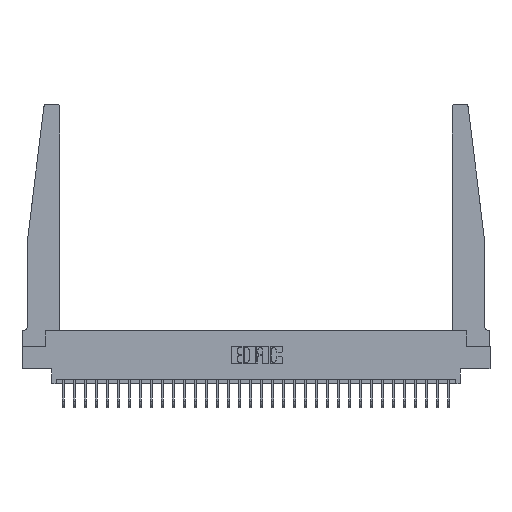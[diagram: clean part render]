
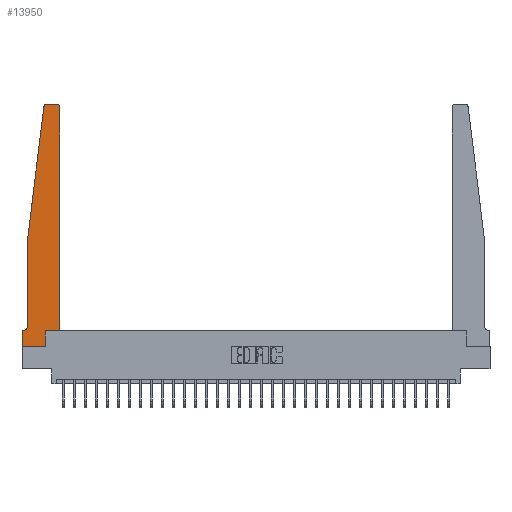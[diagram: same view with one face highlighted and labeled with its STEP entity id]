
A CAD part, top view. The second image highlights one B-rep face of the part: STEP entity #13950.
In plain terms, the highlighted planar face has unit normal (0, 0, 1).
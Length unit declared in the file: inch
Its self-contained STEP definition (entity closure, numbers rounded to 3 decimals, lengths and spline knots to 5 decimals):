
#198 = LINE ( 'NONE', #17417, #5958 ) ;
#226 = LINE ( 'NONE', #15857, #4949 ) ;
#667 = VECTOR ( 'NONE', #9376, 39.37008 ) ;
#750 = CARTESIAN_POINT ( 'NONE',  ( 0.065, 1.25, 0.37 ) ) ;
#854 = CARTESIAN_POINT ( 'NONE',  ( 0.27653, 2.72, 0.37 ) ) ;
#1331 = DIRECTION ( 'NONE',  ( 0., 1., 0. ) ) ;
#1550 = VERTEX_POINT ( 'NONE', #25755 ) ;
#1827 = CIRCLE ( 'NONE', #17989, 0.03 ) ;
#1895 = LINE ( 'NONE', #8431, #2911 ) ;
#2248 = VERTEX_POINT ( 'NONE', #2854 ) ;
#2388 = EDGE_LOOP ( 'NONE', ( #16379, #17962, #22868, #16298, #4187, #12979, #7939, #10421, #23829, #5832, #13279, #14487 ) ) ;
#2640 = AXIS2_PLACEMENT_3D ( 'NONE', #854, #18647, #5355 ) ;
#2854 = CARTESIAN_POINT ( 'NONE',  ( 0.2605, 0.18, 0.37 ) ) ;
#2911 = VECTOR ( 'NONE', #1331, 39.37008 ) ;
#3082 = DIRECTION ( 'NONE',  ( -0.122, -0.992, 0. ) ) ;
#3634 = AXIS2_PLACEMENT_3D ( 'NONE', #10922, #4018, #17439 ) ;
#3909 = EDGE_CURVE ( 'NONE', #10208, #19632, #226, .T. ) ;
#4018 = DIRECTION ( 'NONE',  ( 0., 0., 1. ) ) ;
#4091 = VERTEX_POINT ( 'NONE', #23505 ) ;
#4162 = FACE_OUTER_BOUND ( 'NONE', #2388, .T. ) ;
#4187 = ORIENTED_EDGE ( 'NONE', *, *, #14019, .T. ) ;
#4772 = VERTEX_POINT ( 'NONE', #25900 ) ;
#4949 = VECTOR ( 'NONE', #11215, 39.37008 ) ;
#5355 = DIRECTION ( 'NONE',  ( 1., 0., 0. ) ) ;
#5832 = ORIENTED_EDGE ( 'NONE', *, *, #8914, .T. ) ;
#5921 = VECTOR ( 'NONE', #16745, 39.37008 ) ;
#5958 = VECTOR ( 'NONE', #17986, 39.37008 ) ;
#6301 = VECTOR ( 'NONE', #27481, 39.37008 ) ;
#6758 = DIRECTION ( 'NONE',  ( -1., 0., 0. ) ) ;
#7132 = EDGE_CURVE ( 'NONE', #24352, #4091, #22623, .T. ) ;
#7229 = CARTESIAN_POINT ( 'NONE',  ( 0.015, 0.1875, 0.37 ) ) ;
#7259 = CARTESIAN_POINT ( 'NONE',  ( 0.395, 2.75, 0.37 ) ) ;
#7845 = DIRECTION ( 'NONE',  ( 0., 0., 1. ) ) ;
#7939 = ORIENTED_EDGE ( 'NONE', *, *, #3909, .T. ) ;
#8269 = EDGE_CURVE ( 'NONE', #19632, #15771, #9954, .T. ) ;
#8271 = CARTESIAN_POINT ( 'NONE',  ( 0., 0.1875, 0.37 ) ) ;
#8431 = CARTESIAN_POINT ( 'NONE',  ( 0.425, 0.18, 0.37 ) ) ;
#8697 = VECTOR ( 'NONE', #9607, 39.37008 ) ;
#8860 = CARTESIAN_POINT ( 'NONE',  ( 0.2605, 0., 0.37 ) ) ;
#8914 = EDGE_CURVE ( 'NONE', #2248, #9975, #198, .T. ) ;
#9376 = DIRECTION ( 'NONE',  ( -1., 0., 0. ) ) ;
#9517 = LINE ( 'NONE', #20634, #667 ) ;
#9607 = DIRECTION ( 'NONE',  ( 0., -1., 0. ) ) ;
#9949 = CARTESIAN_POINT ( 'NONE',  ( 0.25, 2.75, 0.37 ) ) ;
#9954 = LINE ( 'NONE', #16896, #21324 ) ;
#9975 = VERTEX_POINT ( 'NONE', #16059 ) ;
#10208 = VERTEX_POINT ( 'NONE', #8271 ) ;
#10421 = ORIENTED_EDGE ( 'NONE', *, *, #8269, .T. ) ;
#10436 = CARTESIAN_POINT ( 'NONE',  ( 0., 0., 0.37 ) ) ;
#10745 = VERTEX_POINT ( 'NONE', #23469 ) ;
#10922 = CARTESIAN_POINT ( 'NONE',  ( 0., 0.1875, 0.37 ) ) ;
#11215 = DIRECTION ( 'NONE',  ( 0., -1., 0. ) ) ;
#12780 = EDGE_CURVE ( 'NONE', #1550, #24352, #15119, .T. ) ;
#12979 = ORIENTED_EDGE ( 'NONE', *, *, #23203, .T. ) ;
#13062 = EDGE_CURVE ( 'NONE', #26908, #1550, #27719, .T. ) ;
#13259 = EDGE_CURVE ( 'NONE', #4091, #10745, #13395, .T. ) ;
#13279 = ORIENTED_EDGE ( 'NONE', *, *, #20565, .T. ) ;
#13395 = LINE ( 'NONE', #750, #8697 ) ;
#13950 = ADVANCED_FACE ( 'NONE', ( #4162 ), #24375, .T. ) ;
#14019 = EDGE_CURVE ( 'NONE', #10745, #27191, #23965, .T. ) ;
#14054 = CARTESIAN_POINT ( 'NONE',  ( 0.065, 1.25, 0.37 ) ) ;
#14487 = ORIENTED_EDGE ( 'NONE', *, *, #15332, .T. ) ;
#15119 = CIRCLE ( 'NONE', #2640, 0.03 ) ;
#15332 = EDGE_CURVE ( 'NONE', #4772, #26908, #1827, .T. ) ;
#15428 = CARTESIAN_POINT ( 'NONE',  ( 0.015, 0.2375, 0.37 ) ) ;
#15771 = VERTEX_POINT ( 'NONE', #8860 ) ;
#15857 = CARTESIAN_POINT ( 'NONE',  ( 0., 0., 0.37 ) ) ;
#16059 = CARTESIAN_POINT ( 'NONE',  ( 0.425, 0.18, 0.37 ) ) ;
#16298 = ORIENTED_EDGE ( 'NONE', *, *, #13259, .T. ) ;
#16379 = ORIENTED_EDGE ( 'NONE', *, *, #13062, .T. ) ;
#16444 = VECTOR ( 'NONE', #3082, 39.37008 ) ;
#16643 = DIRECTION ( 'NONE',  ( 1., 0., 0. ) ) ;
#16745 = DIRECTION ( 'NONE',  ( -1., 0., 0. ) ) ;
#16896 = CARTESIAN_POINT ( 'NONE',  ( 0., 0., 0.37 ) ) ;
#17417 = CARTESIAN_POINT ( 'NONE',  ( 0.425, 0.18, 0.37 ) ) ;
#17439 = DIRECTION ( 'NONE',  ( 1., 0., 0. ) ) ;
#17479 = AXIS2_PLACEMENT_3D ( 'NONE', #15428, #24225, #6758 ) ;
#17962 = ORIENTED_EDGE ( 'NONE', *, *, #12780, .T. ) ;
#17986 = DIRECTION ( 'NONE',  ( 1., 0., 0. ) ) ;
#17989 = AXIS2_PLACEMENT_3D ( 'NONE', #18797, #7845, #16643 ) ;
#18647 = DIRECTION ( 'NONE',  ( 0., 0., 1. ) ) ;
#18660 = CARTESIAN_POINT ( 'NONE',  ( 0.2605, 0.18, 0.37 ) ) ;
#18797 = CARTESIAN_POINT ( 'NONE',  ( 0.395, 2.72, 0.37 ) ) ;
#19632 = VERTEX_POINT ( 'NONE', #10436 ) ;
#20565 = EDGE_CURVE ( 'NONE', #9975, #4772, #1895, .T. ) ;
#20634 = CARTESIAN_POINT ( 'NONE',  ( 0.065, 0.1875, 0.37 ) ) ;
#20834 = LINE ( 'NONE', #18660, #6301 ) ;
#21324 = VECTOR ( 'NONE', #27728, 39.37008 ) ;
#22623 = LINE ( 'NONE', #14054, #16444 ) ;
#22868 = ORIENTED_EDGE ( 'NONE', *, *, #7132, .T. ) ;
#23203 = EDGE_CURVE ( 'NONE', #27191, #10208, #9517, .T. ) ;
#23469 = CARTESIAN_POINT ( 'NONE',  ( 0.065, 0.2375, 0.37 ) ) ;
#23505 = CARTESIAN_POINT ( 'NONE',  ( 0.065, 1.25, 0.37 ) ) ;
#23829 = ORIENTED_EDGE ( 'NONE', *, *, #26992, .T. ) ;
#23965 = CIRCLE ( 'NONE', #17479, 0.05 ) ;
#24225 = DIRECTION ( 'NONE',  ( 0., 0., -1. ) ) ;
#24352 = VERTEX_POINT ( 'NONE', #27952 ) ;
#24375 = PLANE ( 'NONE',  #3634 ) ;
#25755 = CARTESIAN_POINT ( 'NONE',  ( 0.27653, 2.75, 0.37 ) ) ;
#25900 = CARTESIAN_POINT ( 'NONE',  ( 0.425, 2.72, 0.37 ) ) ;
#26908 = VERTEX_POINT ( 'NONE', #7259 ) ;
#26992 = EDGE_CURVE ( 'NONE', #15771, #2248, #20834, .T. ) ;
#27191 = VERTEX_POINT ( 'NONE', #7229 ) ;
#27481 = DIRECTION ( 'NONE',  ( 0., 1., 0. ) ) ;
#27719 = LINE ( 'NONE', #9949, #5921 ) ;
#27728 = DIRECTION ( 'NONE',  ( 1., 0., 0. ) ) ;
#27952 = CARTESIAN_POINT ( 'NONE',  ( 0.24675, 2.72367, 0.37 ) ) ;
